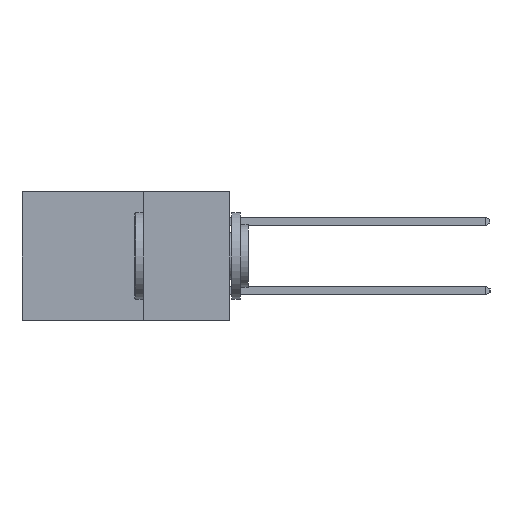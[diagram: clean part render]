
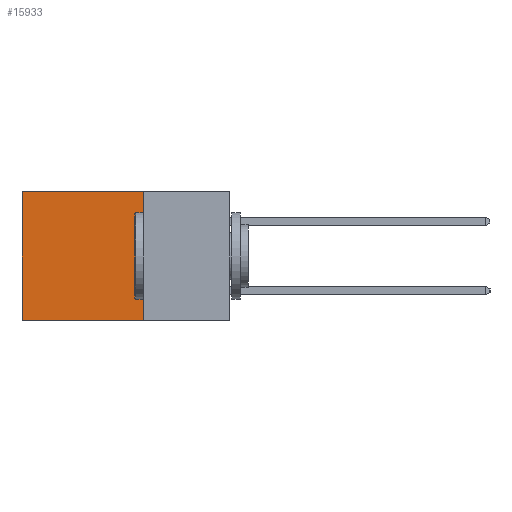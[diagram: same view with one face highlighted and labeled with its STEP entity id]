
A CAD part, left-side view. The second image highlights one B-rep face of the part: STEP entity #15933.
In plain terms, the highlighted planar face has unit normal (-1, 0, 0).
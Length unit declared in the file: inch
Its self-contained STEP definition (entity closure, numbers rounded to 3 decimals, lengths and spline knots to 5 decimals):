
#219 = CARTESIAN_POINT ( 'NONE',  ( 0.2615, 0.6, 0. ) ) ;
#2143 = CARTESIAN_POINT ( 'NONE',  ( 0.2615, 0.6, -0.37 ) ) ;
#3234 = CARTESIAN_POINT ( 'NONE',  ( 0.2615, 0.25, 0. ) ) ;
#3461 = VERTEX_POINT ( 'NONE', #6377 ) ;
#5140 = VECTOR ( 'NONE', #5235, 39.37008 ) ;
#5235 = DIRECTION ( 'NONE',  ( 0., 1., 0. ) ) ;
#5753 = CARTESIAN_POINT ( 'NONE',  ( 0.2615, 0.6, -0.37 ) ) ;
#6029 = VECTOR ( 'NONE', #7830, 39.37008 ) ;
#6377 = CARTESIAN_POINT ( 'NONE',  ( 0.2615, 0.25, 0. ) ) ;
#6692 = LINE ( 'NONE', #5753, #6029 ) ;
#7160 = DIRECTION ( 'NONE',  ( 0., 0., -1. ) ) ;
#7272 = DIRECTION ( 'NONE',  ( 0., 0., -1. ) ) ;
#7830 = DIRECTION ( 'NONE',  ( 0., 0., -1. ) ) ;
#8386 = CARTESIAN_POINT ( 'NONE',  ( 0.2615, 0.25, -0.37 ) ) ;
#8858 = ORIENTED_EDGE ( 'NONE', *, *, #22784, .F. ) ;
#9199 = EDGE_LOOP ( 'NONE', ( #21522, #8858, #23631, #21905 ) ) ;
#10270 = EDGE_CURVE ( 'NONE', #3461, #11429, #15977, .T. ) ;
#10362 = CARTESIAN_POINT ( 'NONE',  ( 0.2615, 0.25, -0.37 ) ) ;
#11331 = CARTESIAN_POINT ( 'NONE',  ( 0.2615, 0.25, -0.37 ) ) ;
#11429 = VERTEX_POINT ( 'NONE', #219 ) ;
#12390 = DIRECTION ( 'NONE',  ( 0., 1., 0. ) ) ;
#12436 = EDGE_CURVE ( 'NONE', #11429, #13341, #6692, .T. ) ;
#13141 = PLANE ( 'NONE',  #18680 ) ;
#13341 = VERTEX_POINT ( 'NONE', #2143 ) ;
#14039 = VECTOR ( 'NONE', #12390, 39.37008 ) ;
#15274 = EDGE_CURVE ( 'NONE', #3461, #16356, #18908, .T. ) ;
#15933 = ADVANCED_FACE ( 'NONE', ( #16361 ), #13141, .F. ) ;
#15977 = LINE ( 'NONE', #3234, #5140 ) ;
#16356 = VERTEX_POINT ( 'NONE', #8386 ) ;
#16361 = FACE_OUTER_BOUND ( 'NONE', #9199, .T. ) ;
#18680 = AXIS2_PLACEMENT_3D ( 'NONE', #23123, #19296, #7160 ) ;
#18908 = LINE ( 'NONE', #11331, #20156 ) ;
#19296 = DIRECTION ( 'NONE',  ( 1., 0., 0. ) ) ;
#19453 = LINE ( 'NONE', #10362, #14039 ) ;
#20156 = VECTOR ( 'NONE', #7272, 39.37008 ) ;
#21522 = ORIENTED_EDGE ( 'NONE', *, *, #12436, .T. ) ;
#21905 = ORIENTED_EDGE ( 'NONE', *, *, #10270, .T. ) ;
#22784 = EDGE_CURVE ( 'NONE', #16356, #13341, #19453, .T. ) ;
#23123 = CARTESIAN_POINT ( 'NONE',  ( 0.2615, 0.25, -0.37 ) ) ;
#23631 = ORIENTED_EDGE ( 'NONE', *, *, #15274, .F. ) ;
